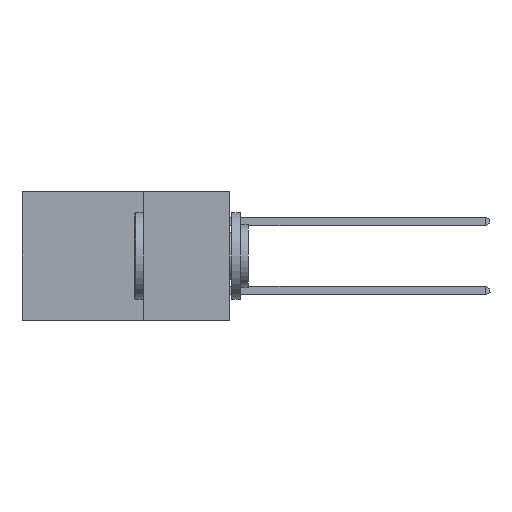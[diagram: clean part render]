
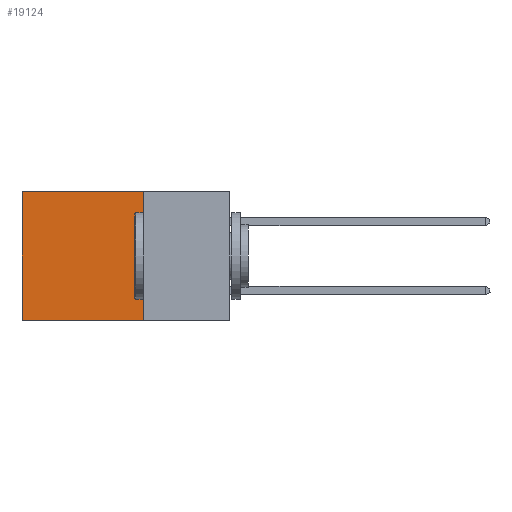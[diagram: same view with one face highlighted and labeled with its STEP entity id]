
A CAD part, left-side view. The second image highlights one B-rep face of the part: STEP entity #19124.
In plain terms, the highlighted planar face has unit normal (-1, 0, 0).
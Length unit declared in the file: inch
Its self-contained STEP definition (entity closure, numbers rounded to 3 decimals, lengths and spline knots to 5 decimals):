
#27 = VECTOR ( 'NONE', #26583, 39.37008 ) ;
#1427 = LINE ( 'NONE', #11219, #27 ) ;
#3111 = LINE ( 'NONE', #7511, #13585 ) ;
#3336 = CARTESIAN_POINT ( 'NONE',  ( 0.298, 0.6, 0. ) ) ;
#5066 = DIRECTION ( 'NONE',  ( 1., 0., 0. ) ) ;
#6208 = CARTESIAN_POINT ( 'NONE',  ( 0.298, 0.25, 0. ) ) ;
#7150 = ORIENTED_EDGE ( 'NONE', *, *, #24163, .F. ) ;
#7510 = VERTEX_POINT ( 'NONE', #3336 ) ;
#7511 = CARTESIAN_POINT ( 'NONE',  ( 0.298, 0.6, 0. ) ) ;
#8349 = VERTEX_POINT ( 'NONE', #17115 ) ;
#8465 = DIRECTION ( 'NONE',  ( 0., 1., 0. ) ) ;
#9036 = CARTESIAN_POINT ( 'NONE',  ( 0.298, 0.25, -0.37 ) ) ;
#9771 = DIRECTION ( 'NONE',  ( 0., 0., -1. ) ) ;
#11219 = CARTESIAN_POINT ( 'NONE',  ( 0.298, 0.25, 0. ) ) ;
#12814 = ORIENTED_EDGE ( 'NONE', *, *, #16248, .T. ) ;
#13157 = AXIS2_PLACEMENT_3D ( 'NONE', #27057, #5066, #20639 ) ;
#13493 = CARTESIAN_POINT ( 'NONE',  ( 0.298, 0.6, -0.37 ) ) ;
#13536 = DIRECTION ( 'NONE',  ( 0., 1., 0. ) ) ;
#13585 = VECTOR ( 'NONE', #9771, 39.37008 ) ;
#15512 = EDGE_CURVE ( 'NONE', #16631, #7510, #27021, .T. ) ;
#15654 = EDGE_CURVE ( 'NONE', #16631, #8349, #1427, .T. ) ;
#16248 = EDGE_CURVE ( 'NONE', #7510, #27454, #3111, .T. ) ;
#16631 = VERTEX_POINT ( 'NONE', #26329 ) ;
#17115 = CARTESIAN_POINT ( 'NONE',  ( 0.298, 0.25, -0.37 ) ) ;
#18389 = PLANE ( 'NONE',  #13157 ) ;
#19124 = ADVANCED_FACE ( 'NONE', ( #26505 ), #18389, .F. ) ;
#19243 = EDGE_LOOP ( 'NONE', ( #12814, #7150, #24743, #19522 ) ) ;
#19522 = ORIENTED_EDGE ( 'NONE', *, *, #15512, .T. ) ;
#20639 = DIRECTION ( 'NONE',  ( 0., 0., -1. ) ) ;
#21188 = VECTOR ( 'NONE', #13536, 39.37008 ) ;
#21268 = VECTOR ( 'NONE', #8465, 39.37008 ) ;
#24163 = EDGE_CURVE ( 'NONE', #8349, #27454, #26941, .T. ) ;
#24743 = ORIENTED_EDGE ( 'NONE', *, *, #15654, .F. ) ;
#26329 = CARTESIAN_POINT ( 'NONE',  ( 0.298, 0.25, 0. ) ) ;
#26505 = FACE_OUTER_BOUND ( 'NONE', #19243, .T. ) ;
#26583 = DIRECTION ( 'NONE',  ( 0., 0., -1. ) ) ;
#26941 = LINE ( 'NONE', #9036, #21188 ) ;
#27021 = LINE ( 'NONE', #6208, #21268 ) ;
#27057 = CARTESIAN_POINT ( 'NONE',  ( 0.298, 0.25, 0. ) ) ;
#27454 = VERTEX_POINT ( 'NONE', #13493 ) ;
